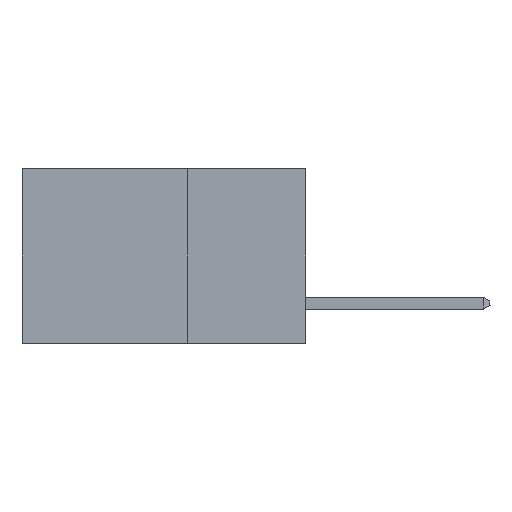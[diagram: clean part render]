
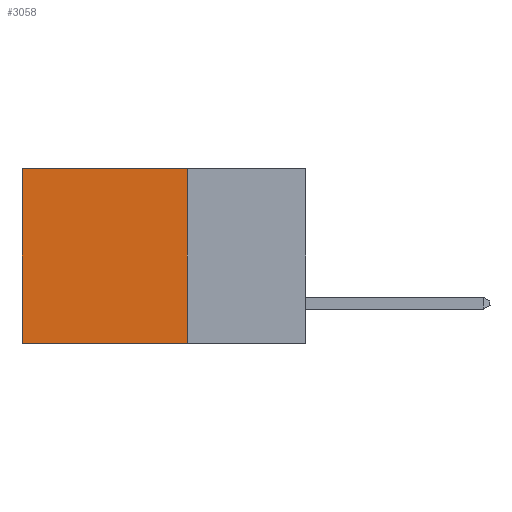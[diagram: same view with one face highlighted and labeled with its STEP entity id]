
A CAD part, left-side view. The second image highlights one B-rep face of the part: STEP entity #3058.
In plain terms, the highlighted planar face has unit normal (-1, 0, 0).
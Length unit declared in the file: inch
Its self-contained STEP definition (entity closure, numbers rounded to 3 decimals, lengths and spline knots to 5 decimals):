
#116 = ORIENTED_EDGE ( 'NONE', *, *, #1474, .T. ) ;
#559 = CARTESIAN_POINT ( 'NONE',  ( 0.298, 0.25, 0. ) ) ;
#623 = FACE_OUTER_BOUND ( 'NONE', #11864, .T. ) ;
#796 = VERTEX_POINT ( 'NONE', #7757 ) ;
#850 = VERTEX_POINT ( 'NONE', #5902 ) ;
#1305 = EDGE_CURVE ( 'NONE', #850, #796, #11962, .T. ) ;
#1374 = ORIENTED_EDGE ( 'NONE', *, *, #12117, .F. ) ;
#1474 = EDGE_CURVE ( 'NONE', #2344, #5676, #7363, .T. ) ;
#2344 = VERTEX_POINT ( 'NONE', #11966 ) ;
#2397 = CARTESIAN_POINT ( 'NONE',  ( 0.298, 0.25, 0. ) ) ;
#2802 = CARTESIAN_POINT ( 'NONE',  ( 0.298, 0.25, -0.37 ) ) ;
#3058 = ADVANCED_FACE ( 'NONE', ( #623 ), #10786, .F. ) ;
#3398 = CARTESIAN_POINT ( 'NONE',  ( 0.298, 0.6, 0. ) ) ;
#4392 = CARTESIAN_POINT ( 'NONE',  ( 0.298, 0.6, 0. ) ) ;
#4478 = DIRECTION ( 'NONE',  ( 0., 0., -1. ) ) ;
#5676 = VERTEX_POINT ( 'NONE', #4392 ) ;
#5739 = CARTESIAN_POINT ( 'NONE',  ( 0.298, 0.25, 0. ) ) ;
#5902 = CARTESIAN_POINT ( 'NONE',  ( 0.298, 0.25, -0.37 ) ) ;
#6463 = AXIS2_PLACEMENT_3D ( 'NONE', #2397, #9013, #11060 ) ;
#6494 = ORIENTED_EDGE ( 'NONE', *, *, #1305, .F. ) ;
#6623 = DIRECTION ( 'NONE',  ( 0., 0., -1. ) ) ;
#6787 = VECTOR ( 'NONE', #9700, 39.37008 ) ;
#7363 = LINE ( 'NONE', #559, #8113 ) ;
#7757 = CARTESIAN_POINT ( 'NONE',  ( 0.298, 0.6, -0.37 ) ) ;
#8113 = VECTOR ( 'NONE', #11852, 39.37008 ) ;
#8607 = LINE ( 'NONE', #5739, #11246 ) ;
#9013 = DIRECTION ( 'NONE',  ( 1., 0., 0. ) ) ;
#9700 = DIRECTION ( 'NONE',  ( 0., 1., 0. ) ) ;
#10044 = ORIENTED_EDGE ( 'NONE', *, *, #11051, .T. ) ;
#10786 = PLANE ( 'NONE',  #6463 ) ;
#11051 = EDGE_CURVE ( 'NONE', #5676, #796, #11590, .T. ) ;
#11060 = DIRECTION ( 'NONE',  ( 0., 0., -1. ) ) ;
#11246 = VECTOR ( 'NONE', #6623, 39.37008 ) ;
#11590 = LINE ( 'NONE', #3398, #11727 ) ;
#11727 = VECTOR ( 'NONE', #4478, 39.37008 ) ;
#11852 = DIRECTION ( 'NONE',  ( 0., 1., 0. ) ) ;
#11864 = EDGE_LOOP ( 'NONE', ( #10044, #6494, #1374, #116 ) ) ;
#11962 = LINE ( 'NONE', #2802, #6787 ) ;
#11966 = CARTESIAN_POINT ( 'NONE',  ( 0.298, 0.25, 0. ) ) ;
#12117 = EDGE_CURVE ( 'NONE', #2344, #850, #8607, .T. ) ;
